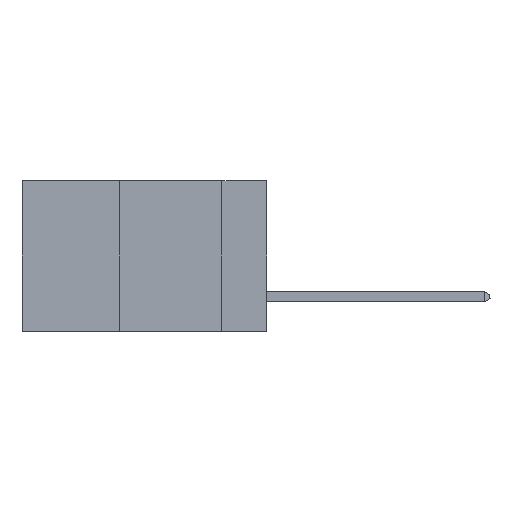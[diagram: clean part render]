
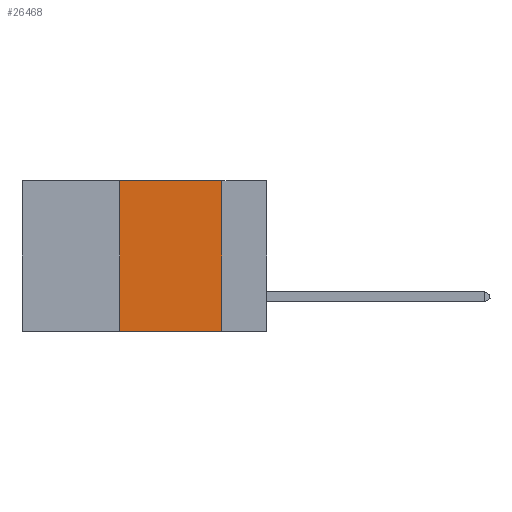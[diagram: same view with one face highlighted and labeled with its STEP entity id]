
A CAD part, left-side view. The second image highlights one B-rep face of the part: STEP entity #26468.
In plain terms, the highlighted planar face has unit normal (-1, 0, 0).
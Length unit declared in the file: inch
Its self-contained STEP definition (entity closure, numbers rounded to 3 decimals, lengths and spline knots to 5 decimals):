
#358 = VECTOR ( 'NONE', #19345, 39.37008 ) ;
#1480 = EDGE_CURVE ( 'NONE', #2367, #18699, #25177, .T. ) ;
#2055 = ORIENTED_EDGE ( 'NONE', *, *, #15806, .F. ) ;
#2367 = VERTEX_POINT ( 'NONE', #14437 ) ;
#2480 = LINE ( 'NONE', #22475, #8096 ) ;
#4029 = VERTEX_POINT ( 'NONE', #15787 ) ;
#4327 = DIRECTION ( 'NONE',  ( 1., 0., 0. ) ) ;
#4418 = CARTESIAN_POINT ( 'NONE',  ( 0., 0.6, 0. ) ) ;
#4881 = EDGE_CURVE ( 'NONE', #4029, #2367, #2480, .T. ) ;
#5870 = ORIENTED_EDGE ( 'NONE', *, *, #19567, .T. ) ;
#5981 = LINE ( 'NONE', #17358, #358 ) ;
#6325 = VECTOR ( 'NONE', #26035, 39.37008 ) ;
#8096 = VECTOR ( 'NONE', #26718, 39.37008 ) ;
#9833 = VERTEX_POINT ( 'NONE', #22857 ) ;
#10140 = AXIS2_PLACEMENT_3D ( 'NONE', #4418, #4327, #19195 ) ;
#12700 = ORIENTED_EDGE ( 'NONE', *, *, #4881, .F. ) ;
#12865 = FACE_OUTER_BOUND ( 'NONE', #26949, .T. ) ;
#13535 = CARTESIAN_POINT ( 'NONE',  ( 0., 0.6, -0.37 ) ) ;
#14437 = CARTESIAN_POINT ( 'NONE',  ( 0., 0.36, 0. ) ) ;
#15787 = CARTESIAN_POINT ( 'NONE',  ( 0., 0.36, -0.37 ) ) ;
#15806 = EDGE_CURVE ( 'NONE', #18699, #9833, #5981, .T. ) ;
#17358 = CARTESIAN_POINT ( 'NONE',  ( 0., 0.11, 0. ) ) ;
#17771 = ORIENTED_EDGE ( 'NONE', *, *, #1480, .F. ) ;
#18212 = DIRECTION ( 'NONE',  ( 0., -1., 0. ) ) ;
#18699 = VERTEX_POINT ( 'NONE', #21013 ) ;
#18737 = LINE ( 'NONE', #13535, #26032 ) ;
#19195 = DIRECTION ( 'NONE',  ( 0., 0., -1. ) ) ;
#19345 = DIRECTION ( 'NONE',  ( 0., 0., -1. ) ) ;
#19567 = EDGE_CURVE ( 'NONE', #4029, #9833, #18737, .T. ) ;
#21013 = CARTESIAN_POINT ( 'NONE',  ( 0., 0.11, 0. ) ) ;
#21526 = PLANE ( 'NONE',  #10140 ) ;
#22475 = CARTESIAN_POINT ( 'NONE',  ( 0., 0.36, 0. ) ) ;
#22857 = CARTESIAN_POINT ( 'NONE',  ( 0., 0.11, -0.37 ) ) ;
#23635 = CARTESIAN_POINT ( 'NONE',  ( 0., 0.6, 0. ) ) ;
#25177 = LINE ( 'NONE', #23635, #6325 ) ;
#26032 = VECTOR ( 'NONE', #18212, 39.37008 ) ;
#26035 = DIRECTION ( 'NONE',  ( 0., -1., 0. ) ) ;
#26468 = ADVANCED_FACE ( 'NONE', ( #12865 ), #21526, .F. ) ;
#26718 = DIRECTION ( 'NONE',  ( 0., 0., 1. ) ) ;
#26949 = EDGE_LOOP ( 'NONE', ( #2055, #17771, #12700, #5870 ) ) ;
